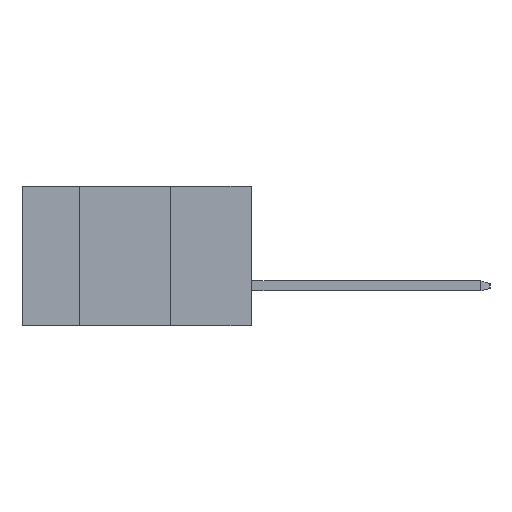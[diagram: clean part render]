
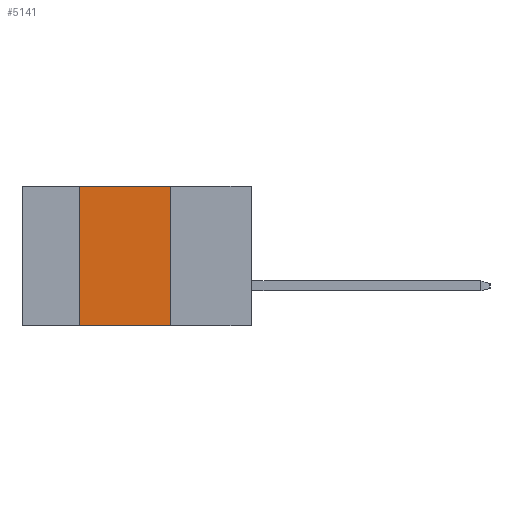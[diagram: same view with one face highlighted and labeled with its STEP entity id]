
A CAD part, left-side view. The second image highlights one B-rep face of the part: STEP entity #5141.
In plain terms, the highlighted planar face has unit normal (-1, 0, 0).
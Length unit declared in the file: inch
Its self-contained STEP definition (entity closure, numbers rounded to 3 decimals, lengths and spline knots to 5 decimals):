
#196 = ORIENTED_EDGE ( 'NONE', *, *, #9661, .F. ) ;
#285 = CARTESIAN_POINT ( 'NONE',  ( 0., 0.54, -0.437 ) ) ;
#721 = VECTOR ( 'NONE', #7611, 39.37008 ) ;
#1347 = VERTEX_POINT ( 'NONE', #9004 ) ;
#1890 = CARTESIAN_POINT ( 'NONE',  ( 0., 0.254, -0.437 ) ) ;
#1945 = LINE ( 'NONE', #9803, #8615 ) ;
#2124 = CARTESIAN_POINT ( 'NONE',  ( 0., 0.72, 0. ) ) ;
#2514 = VERTEX_POINT ( 'NONE', #285 ) ;
#2692 = DIRECTION ( 'NONE',  ( 0., -1., 0. ) ) ;
#2696 = ORIENTED_EDGE ( 'NONE', *, *, #7103, .F. ) ;
#2714 = EDGE_CURVE ( 'NONE', #4500, #1347, #3580, .T. ) ;
#2804 = ORIENTED_EDGE ( 'NONE', *, *, #3023, .T. ) ;
#3023 = EDGE_CURVE ( 'NONE', #2514, #6757, #8798, .T. ) ;
#3080 = LINE ( 'NONE', #6222, #5804 ) ;
#3210 = EDGE_LOOP ( 'NONE', ( #2696, #8379, #196, #2804 ) ) ;
#3580 = LINE ( 'NONE', #2124, #721 ) ;
#4427 = PLANE ( 'NONE',  #5592 ) ;
#4500 = VERTEX_POINT ( 'NONE', #7761 ) ;
#4727 = DIRECTION ( 'NONE',  ( 0., 0., -1. ) ) ;
#5141 = ADVANCED_FACE ( 'NONE', ( #9179 ), #4427, .F. ) ;
#5145 = CARTESIAN_POINT ( 'NONE',  ( 0., 0.72, 0. ) ) ;
#5491 = VECTOR ( 'NONE', #2692, 39.37008 ) ;
#5592 = AXIS2_PLACEMENT_3D ( 'NONE', #5145, #6653, #8310 ) ;
#5804 = VECTOR ( 'NONE', #4727, 39.37008 ) ;
#6222 = CARTESIAN_POINT ( 'NONE',  ( 0., 0.254, -0.437 ) ) ;
#6653 = DIRECTION ( 'NONE',  ( 1., 0., 0. ) ) ;
#6757 = VERTEX_POINT ( 'NONE', #1890 ) ;
#7103 = EDGE_CURVE ( 'NONE', #1347, #6757, #3080, .T. ) ;
#7611 = DIRECTION ( 'NONE',  ( 0., -1., 0. ) ) ;
#7761 = CARTESIAN_POINT ( 'NONE',  ( 0., 0.54, 0. ) ) ;
#8310 = DIRECTION ( 'NONE',  ( 0., 0., -1. ) ) ;
#8379 = ORIENTED_EDGE ( 'NONE', *, *, #2714, .F. ) ;
#8615 = VECTOR ( 'NONE', #9081, 39.37008 ) ;
#8798 = LINE ( 'NONE', #9769, #5491 ) ;
#9004 = CARTESIAN_POINT ( 'NONE',  ( 0., 0.254, 0. ) ) ;
#9081 = DIRECTION ( 'NONE',  ( 0., 0., 1. ) ) ;
#9179 = FACE_OUTER_BOUND ( 'NONE', #3210, .T. ) ;
#9661 = EDGE_CURVE ( 'NONE', #2514, #4500, #1945, .T. ) ;
#9769 = CARTESIAN_POINT ( 'NONE',  ( 0., 0.72, -0.437 ) ) ;
#9803 = CARTESIAN_POINT ( 'NONE',  ( 0., 0.54, -0.437 ) ) ;
